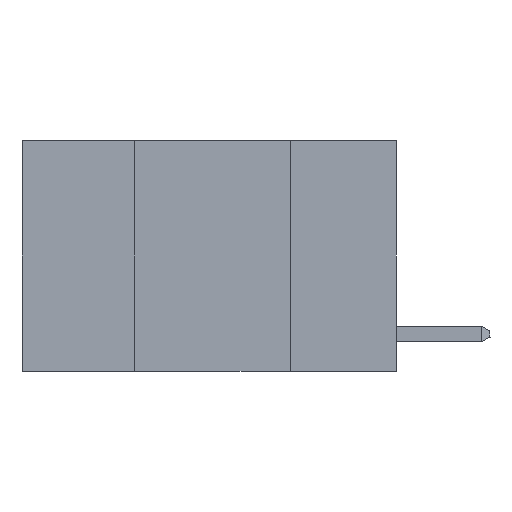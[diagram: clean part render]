
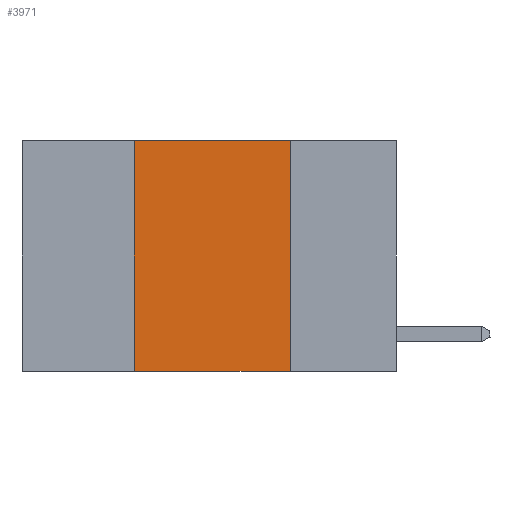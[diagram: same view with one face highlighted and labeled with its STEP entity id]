
A CAD part, left-side view. The second image highlights one B-rep face of the part: STEP entity #3971.
In plain terms, the highlighted planar face has unit normal (-1, 0, 0).
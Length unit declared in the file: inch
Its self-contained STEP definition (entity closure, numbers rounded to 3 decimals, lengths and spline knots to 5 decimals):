
#49 = LINE ( 'NONE', #5974, #4587 ) ;
#145 = FACE_OUTER_BOUND ( 'NONE', #11525, .T. ) ;
#425 = DIRECTION ( 'NONE',  ( 1., 0., 0. ) ) ;
#684 = CARTESIAN_POINT ( 'NONE',  ( 0., 0.42, 0. ) ) ;
#848 = DIRECTION ( 'NONE',  ( 0., 0., -1. ) ) ;
#1127 = PLANE ( 'NONE',  #7007 ) ;
#1296 = CARTESIAN_POINT ( 'NONE',  ( 0., 0.6, 0. ) ) ;
#1418 = CARTESIAN_POINT ( 'NONE',  ( 0., 0.17, -0.37 ) ) ;
#1877 = CARTESIAN_POINT ( 'NONE',  ( 0., 0.6, 0. ) ) ;
#2088 = ORIENTED_EDGE ( 'NONE', *, *, #8281, .F. ) ;
#2335 = VECTOR ( 'NONE', #5764, 39.37008 ) ;
#2442 = ORIENTED_EDGE ( 'NONE', *, *, #8468, .F. ) ;
#2475 = VERTEX_POINT ( 'NONE', #7791 ) ;
#3885 = CARTESIAN_POINT ( 'NONE',  ( 0., 0.6, -0.37 ) ) ;
#3971 = ADVANCED_FACE ( 'NONE', ( #145 ), #1127, .F. ) ;
#4138 = ORIENTED_EDGE ( 'NONE', *, *, #9947, .F. ) ;
#4271 = VECTOR ( 'NONE', #4913, 39.37008 ) ;
#4571 = LINE ( 'NONE', #1296, #4271 ) ;
#4587 = VECTOR ( 'NONE', #6900, 39.37008 ) ;
#4810 = CARTESIAN_POINT ( 'NONE',  ( 0., 0.17, 0. ) ) ;
#4913 = DIRECTION ( 'NONE',  ( 0., -1., 0. ) ) ;
#5764 = DIRECTION ( 'NONE',  ( 0., 0., -1. ) ) ;
#5796 = ORIENTED_EDGE ( 'NONE', *, *, #10417, .T. ) ;
#5974 = CARTESIAN_POINT ( 'NONE',  ( 0., 0.42, 0. ) ) ;
#6872 = VERTEX_POINT ( 'NONE', #1418 ) ;
#6900 = DIRECTION ( 'NONE',  ( 0., 0., 1. ) ) ;
#7007 = AXIS2_PLACEMENT_3D ( 'NONE', #1877, #425, #848 ) ;
#7791 = CARTESIAN_POINT ( 'NONE',  ( 0., 0.42, -0.37 ) ) ;
#7951 = CARTESIAN_POINT ( 'NONE',  ( 0., 0.17, 0. ) ) ;
#8281 = EDGE_CURVE ( 'NONE', #9111, #6872, #9027, .T. ) ;
#8468 = EDGE_CURVE ( 'NONE', #2475, #10095, #49, .T. ) ;
#9027 = LINE ( 'NONE', #4810, #2335 ) ;
#9111 = VERTEX_POINT ( 'NONE', #7951 ) ;
#9270 = LINE ( 'NONE', #3885, #9824 ) ;
#9824 = VECTOR ( 'NONE', #11125, 39.37008 ) ;
#9947 = EDGE_CURVE ( 'NONE', #10095, #9111, #4571, .T. ) ;
#10095 = VERTEX_POINT ( 'NONE', #684 ) ;
#10417 = EDGE_CURVE ( 'NONE', #2475, #6872, #9270, .T. ) ;
#11125 = DIRECTION ( 'NONE',  ( 0., -1., 0. ) ) ;
#11525 = EDGE_LOOP ( 'NONE', ( #2088, #4138, #2442, #5796 ) ) ;
